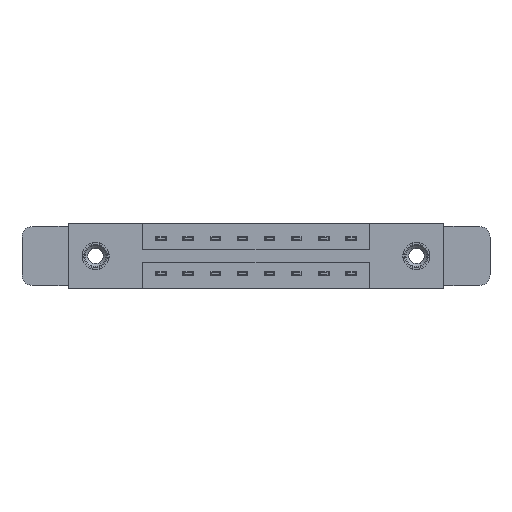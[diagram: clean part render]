
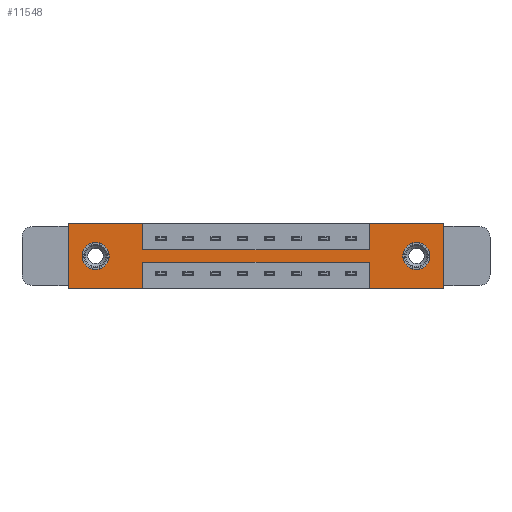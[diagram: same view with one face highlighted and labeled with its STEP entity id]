
A CAD part, front view. The second image highlights one B-rep face of the part: STEP entity #11548.
In plain terms, the highlighted planar face has unit normal (0, -1, 0).
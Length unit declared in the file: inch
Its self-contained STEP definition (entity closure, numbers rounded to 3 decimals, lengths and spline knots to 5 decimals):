
#37 = AXIS2_PLACEMENT_3D ( 'NONE', #1679, #2565, #2608 ) ;
#143 = FACE_OUTER_BOUND ( 'NONE', #8605, .T. ) ;
#300 = VERTEX_POINT ( 'NONE', #7859 ) ;
#388 = ORIENTED_EDGE ( 'NONE', *, *, #4852, .F. ) ;
#542 = DIRECTION ( 'NONE',  ( 1., 0., 0. ) ) ;
#590 = EDGE_CURVE ( 'NONE', #3565, #7974, #2676, .T. ) ;
#694 = DIRECTION ( 'NONE',  ( 0., 1., 0. ) ) ;
#771 = DIRECTION ( 'NONE',  ( -1., 0., 0. ) ) ;
#856 = CARTESIAN_POINT ( 'NONE',  ( 0., 0., -0.37 ) ) ;
#1007 = DIRECTION ( 'NONE',  ( -1., 0., 0. ) ) ;
#1142 = EDGE_CURVE ( 'NONE', #11742, #9750, #3440, .T. ) ;
#1176 = CARTESIAN_POINT ( 'NONE',  ( 1.729, 0., 0. ) ) ;
#1422 = LINE ( 'NONE', #7082, #12623 ) ;
#1679 = CARTESIAN_POINT ( 'NONE',  ( 0., 0., -0.37 ) ) ;
#1954 = VERTEX_POINT ( 'NONE', #4486 ) ;
#2076 = FACE_BOUND ( 'NONE', #5233, .T. ) ;
#2079 = LINE ( 'NONE', #3416, #8328 ) ;
#2259 = VECTOR ( 'NONE', #11729, 39.37008 ) ;
#2374 = DIRECTION ( 'NONE',  ( 0., 1., 0. ) ) ;
#2506 = CARTESIAN_POINT ( 'NONE',  ( 0.155, 0., -0.185 ) ) ;
#2565 = DIRECTION ( 'NONE',  ( 0., -1., 0. ) ) ;
#2608 = DIRECTION ( 'NONE',  ( 0., 0., -1. ) ) ;
#2676 = LINE ( 'NONE', #11275, #5200 ) ;
#2682 = CARTESIAN_POINT ( 'NONE',  ( 1.999, 0., -0.107 ) ) ;
#2948 = CARTESIAN_POINT ( 'NONE',  ( 0., 0., 0. ) ) ;
#3075 = CARTESIAN_POINT ( 'NONE',  ( 2.154, 0., -0.37 ) ) ;
#3167 = DIRECTION ( 'NONE',  ( -1., 0., 0. ) ) ;
#3416 = CARTESIAN_POINT ( 'NONE',  ( 1.729, 0., 0. ) ) ;
#3440 = LINE ( 'NONE', #6134, #10491 ) ;
#3565 = VERTEX_POINT ( 'NONE', #1176 ) ;
#3671 = EDGE_CURVE ( 'NONE', #7686, #11742, #10758, .T. ) ;
#3725 = VERTEX_POINT ( 'NONE', #6493 ) ;
#3907 = EDGE_CURVE ( 'NONE', #3725, #11045, #11695, .T. ) ;
#4157 = CARTESIAN_POINT ( 'NONE',  ( 0.425, 0., -0.15 ) ) ;
#4183 = EDGE_CURVE ( 'NONE', #7974, #12101, #10270, .T. ) ;
#4337 = DIRECTION ( 'NONE',  ( 1., 0., 0. ) ) ;
#4397 = ORIENTED_EDGE ( 'NONE', *, *, #12487, .F. ) ;
#4446 = CIRCLE ( 'NONE', #5190, 0.078 ) ;
#4486 = CARTESIAN_POINT ( 'NONE',  ( 0.155, 0., -0.263 ) ) ;
#4657 = AXIS2_PLACEMENT_3D ( 'NONE', #12438, #2374, #7485 ) ;
#4785 = DIRECTION ( 'NONE',  ( 0., 0., -1. ) ) ;
#4852 = EDGE_CURVE ( 'NONE', #12840, #7686, #9431, .T. ) ;
#4879 = VECTOR ( 'NONE', #771, 39.37008 ) ;
#5190 = AXIS2_PLACEMENT_3D ( 'NONE', #9370, #7528, #4785 ) ;
#5200 = VECTOR ( 'NONE', #4337, 39.37008 ) ;
#5233 = EDGE_LOOP ( 'NONE', ( #7498, #9692 ) ) ;
#5429 = CARTESIAN_POINT ( 'NONE',  ( 0.425, 0., -0.37 ) ) ;
#5517 = ORIENTED_EDGE ( 'NONE', *, *, #10443, .F. ) ;
#5521 = FACE_BOUND ( 'NONE', #6539, .T. ) ;
#5580 = DIRECTION ( 'NONE',  ( 0., 0., 1. ) ) ;
#5789 = ORIENTED_EDGE ( 'NONE', *, *, #590, .F. ) ;
#5797 = EDGE_CURVE ( 'NONE', #11045, #12840, #1422, .T. ) ;
#5958 = VERTEX_POINT ( 'NONE', #6309 ) ;
#5983 = ORIENTED_EDGE ( 'NONE', *, *, #6053, .F. ) ;
#5989 = LINE ( 'NONE', #4157, #8812 ) ;
#6053 = EDGE_CURVE ( 'NONE', #12159, #3565, #2079, .T. ) ;
#6134 = CARTESIAN_POINT ( 'NONE',  ( 0.425, 0., 0. ) ) ;
#6156 = CARTESIAN_POINT ( 'NONE',  ( 2.154, 0., 0. ) ) ;
#6224 = CARTESIAN_POINT ( 'NONE',  ( 1.729, 0., -0.22 ) ) ;
#6283 = LINE ( 'NONE', #10339, #10697 ) ;
#6309 = CARTESIAN_POINT ( 'NONE',  ( 1.999, 0., -0.263 ) ) ;
#6361 = EDGE_CURVE ( 'NONE', #300, #10192, #6283, .T. ) ;
#6493 = CARTESIAN_POINT ( 'NONE',  ( 0.425, 0., -0.22 ) ) ;
#6539 = EDGE_LOOP ( 'NONE', ( #7217, #7480 ) ) ;
#7001 = ORIENTED_EDGE ( 'NONE', *, *, #4183, .F. ) ;
#7082 = CARTESIAN_POINT ( 'NONE',  ( 0., 0., -0.37 ) ) ;
#7185 = DIRECTION ( 'NONE',  ( 1., 0., 0. ) ) ;
#7189 = VERTEX_POINT ( 'NONE', #12875 ) ;
#7192 = CARTESIAN_POINT ( 'NONE',  ( 0.425, 0., 0. ) ) ;
#7217 = ORIENTED_EDGE ( 'NONE', *, *, #8003, .T. ) ;
#7480 = ORIENTED_EDGE ( 'NONE', *, *, #8153, .T. ) ;
#7485 = DIRECTION ( 'NONE',  ( 0., 0., 1. ) ) ;
#7498 = ORIENTED_EDGE ( 'NONE', *, *, #10892, .T. ) ;
#7528 = DIRECTION ( 'NONE',  ( 0., 1., 0. ) ) ;
#7564 = CARTESIAN_POINT ( 'NONE',  ( 0.425, 0., -0.37 ) ) ;
#7686 = VERTEX_POINT ( 'NONE', #2948 ) ;
#7694 = ORIENTED_EDGE ( 'NONE', *, *, #5797, .F. ) ;
#7769 = CIRCLE ( 'NONE', #10452, 0.078 ) ;
#7825 = LINE ( 'NONE', #8142, #10344 ) ;
#7859 = CARTESIAN_POINT ( 'NONE',  ( 1.729, 0., -0.37 ) ) ;
#7974 = VERTEX_POINT ( 'NONE', #8407 ) ;
#8003 = EDGE_CURVE ( 'NONE', #7189, #1954, #8390, .T. ) ;
#8068 = VECTOR ( 'NONE', #542, 39.37008 ) ;
#8142 = CARTESIAN_POINT ( 'NONE',  ( 0., 0., -0.37 ) ) ;
#8153 = EDGE_CURVE ( 'NONE', #1954, #7189, #7769, .T. ) ;
#8260 = AXIS2_PLACEMENT_3D ( 'NONE', #12257, #9192, #10235 ) ;
#8293 = LINE ( 'NONE', #11813, #4879 ) ;
#8328 = VECTOR ( 'NONE', #5580, 39.37008 ) ;
#8390 = CIRCLE ( 'NONE', #4657, 0.078 ) ;
#8399 = CARTESIAN_POINT ( 'NONE',  ( 0., 0., 0. ) ) ;
#8407 = CARTESIAN_POINT ( 'NONE',  ( 2.154, 0., 0. ) ) ;
#8605 = EDGE_LOOP ( 'NONE', ( #10937, #9885, #12392, #4397, #7001, #5789, #5983, #5517, #12252, #9297, #388, #7694 ) ) ;
#8640 = CARTESIAN_POINT ( 'NONE',  ( 0.425, 0., -0.15 ) ) ;
#8812 = VECTOR ( 'NONE', #7185, 39.37008 ) ;
#8902 = DIRECTION ( 'NONE',  ( 0., 0., 1. ) ) ;
#9192 = DIRECTION ( 'NONE',  ( 0., 1., 0. ) ) ;
#9297 = ORIENTED_EDGE ( 'NONE', *, *, #3671, .F. ) ;
#9370 = CARTESIAN_POINT ( 'NONE',  ( 1.999, 0., -0.185 ) ) ;
#9431 = LINE ( 'NONE', #9829, #9757 ) ;
#9534 = EDGE_CURVE ( 'NONE', #5958, #12551, #4446, .T. ) ;
#9692 = ORIENTED_EDGE ( 'NONE', *, *, #9534, .T. ) ;
#9750 = VERTEX_POINT ( 'NONE', #8640 ) ;
#9757 = VECTOR ( 'NONE', #8902, 39.37008 ) ;
#9829 = CARTESIAN_POINT ( 'NONE',  ( 0., 0., 0. ) ) ;
#9885 = ORIENTED_EDGE ( 'NONE', *, *, #12068, .F. ) ;
#10192 = VERTEX_POINT ( 'NONE', #6224 ) ;
#10235 = DIRECTION ( 'NONE',  ( 0., 0., -1. ) ) ;
#10270 = LINE ( 'NONE', #6156, #2259 ) ;
#10339 = CARTESIAN_POINT ( 'NONE',  ( 1.729, 0., -0.37 ) ) ;
#10344 = VECTOR ( 'NONE', #1007, 39.37008 ) ;
#10443 = EDGE_CURVE ( 'NONE', #9750, #12159, #5989, .T. ) ;
#10452 = AXIS2_PLACEMENT_3D ( 'NONE', #2506, #694, #11586 ) ;
#10491 = VECTOR ( 'NONE', #11099, 39.37008 ) ;
#10493 = CARTESIAN_POINT ( 'NONE',  ( 1.729, 0., -0.15 ) ) ;
#10697 = VECTOR ( 'NONE', #12332, 39.37008 ) ;
#10758 = LINE ( 'NONE', #8399, #8068 ) ;
#10892 = EDGE_CURVE ( 'NONE', #12551, #5958, #11667, .T. ) ;
#10937 = ORIENTED_EDGE ( 'NONE', *, *, #3907, .F. ) ;
#11045 = VERTEX_POINT ( 'NONE', #7564 ) ;
#11099 = DIRECTION ( 'NONE',  ( 0., 0., -1. ) ) ;
#11275 = CARTESIAN_POINT ( 'NONE',  ( 0., 0., 0. ) ) ;
#11368 = VECTOR ( 'NONE', #12456, 39.37008 ) ;
#11548 = ADVANCED_FACE ( 'NONE', ( #2076, #5521, #143 ), #12727, .T. ) ;
#11586 = DIRECTION ( 'NONE',  ( 0., 0., 1. ) ) ;
#11667 = CIRCLE ( 'NONE', #8260, 0.078 ) ;
#11695 = LINE ( 'NONE', #5429, #11368 ) ;
#11729 = DIRECTION ( 'NONE',  ( 0., 0., -1. ) ) ;
#11742 = VERTEX_POINT ( 'NONE', #7192 ) ;
#11813 = CARTESIAN_POINT ( 'NONE',  ( 0.425, 0., -0.22 ) ) ;
#12068 = EDGE_CURVE ( 'NONE', #10192, #3725, #8293, .T. ) ;
#12101 = VERTEX_POINT ( 'NONE', #3075 ) ;
#12159 = VERTEX_POINT ( 'NONE', #10493 ) ;
#12252 = ORIENTED_EDGE ( 'NONE', *, *, #1142, .F. ) ;
#12257 = CARTESIAN_POINT ( 'NONE',  ( 1.999, 0., -0.185 ) ) ;
#12332 = DIRECTION ( 'NONE',  ( 0., 0., 1. ) ) ;
#12392 = ORIENTED_EDGE ( 'NONE', *, *, #6361, .F. ) ;
#12438 = CARTESIAN_POINT ( 'NONE',  ( 0.155, 0., -0.185 ) ) ;
#12456 = DIRECTION ( 'NONE',  ( 0., 0., -1. ) ) ;
#12487 = EDGE_CURVE ( 'NONE', #12101, #300, #7825, .T. ) ;
#12551 = VERTEX_POINT ( 'NONE', #2682 ) ;
#12623 = VECTOR ( 'NONE', #3167, 39.37008 ) ;
#12727 = PLANE ( 'NONE',  #37 ) ;
#12840 = VERTEX_POINT ( 'NONE', #856 ) ;
#12875 = CARTESIAN_POINT ( 'NONE',  ( 0.155, 0., -0.107 ) ) ;
